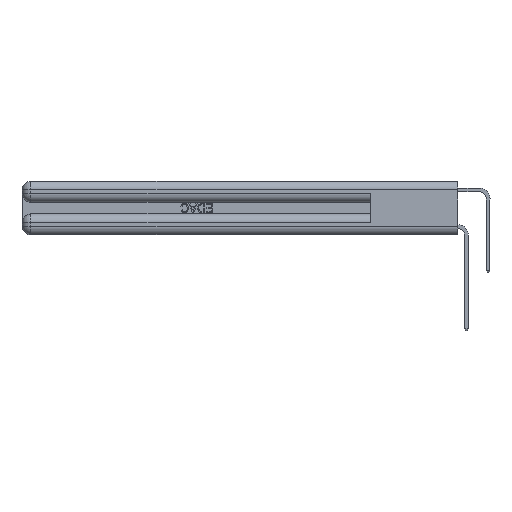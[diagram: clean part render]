
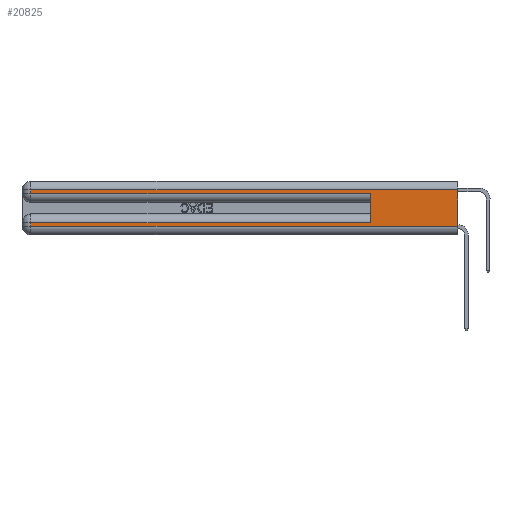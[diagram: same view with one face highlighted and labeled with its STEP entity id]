
A CAD part, left-side view. The second image highlights one B-rep face of the part: STEP entity #20825.
In plain terms, the highlighted planar face has unit normal (-1, 0, 0).
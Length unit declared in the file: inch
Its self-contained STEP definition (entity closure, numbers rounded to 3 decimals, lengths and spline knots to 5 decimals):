
#70 = LINE ( 'NONE', #30249, #3659 ) ;
#272 = DIRECTION ( 'NONE',  ( 0., 0., -1. ) ) ;
#492 = CARTESIAN_POINT ( 'NONE',  ( 0., 0., 0.37 ) ) ;
#1123 = LINE ( 'NONE', #13394, #12926 ) ;
#1516 = VECTOR ( 'NONE', #16111, 39.37008 ) ;
#1933 = CARTESIAN_POINT ( 'NONE',  ( 0., 0., 0.285 ) ) ;
#1957 = CARTESIAN_POINT ( 'NONE',  ( 0., 0., 0.37 ) ) ;
#2993 = DIRECTION ( 'NONE',  ( 0., 0., 1. ) ) ;
#3484 = CARTESIAN_POINT ( 'NONE',  ( 0., 0., 0.31 ) ) ;
#3612 = CARTESIAN_POINT ( 'NONE',  ( 0., 0., 0.06 ) ) ;
#3659 = VECTOR ( 'NONE', #2993, 39.37008 ) ;
#4809 = VECTOR ( 'NONE', #12495, 39.37008 ) ;
#4818 = EDGE_CURVE ( 'NONE', #23546, #12171, #24266, .T. ) ;
#5651 = VECTOR ( 'NONE', #6399, 39.37008 ) ;
#6399 = DIRECTION ( 'NONE',  ( 0., 1., 0. ) ) ;
#8438 = EDGE_CURVE ( 'NONE', #11112, #12171, #9797, .T. ) ;
#8594 = CARTESIAN_POINT ( 'NONE',  ( 0., 2.94, 0.37 ) ) ;
#9797 = LINE ( 'NONE', #31076, #1516 ) ;
#10317 = DIRECTION ( 'NONE',  ( 0., 1., 0. ) ) ;
#10382 = ORIENTED_EDGE ( 'NONE', *, *, #24543, .T. ) ;
#10434 = VECTOR ( 'NONE', #10317, 39.37008 ) ;
#10583 = AXIS2_PLACEMENT_3D ( 'NONE', #1957, #25064, #27660 ) ;
#11105 = DIRECTION ( 'NONE',  ( 0., 0., -1. ) ) ;
#11112 = VERTEX_POINT ( 'NONE', #29518 ) ;
#12127 = ORIENTED_EDGE ( 'NONE', *, *, #8438, .T. ) ;
#12171 = VERTEX_POINT ( 'NONE', #3612 ) ;
#12495 = DIRECTION ( 'NONE',  ( 0., -1., 0. ) ) ;
#12529 = VERTEX_POINT ( 'NONE', #23239 ) ;
#12844 = CARTESIAN_POINT ( 'NONE',  ( 0., 0., 0.31 ) ) ;
#12926 = VECTOR ( 'NONE', #20945, 39.37008 ) ;
#13193 = LINE ( 'NONE', #31609, #5651 ) ;
#13394 = CARTESIAN_POINT ( 'NONE',  ( 0., 2.94, 0.37 ) ) ;
#13824 = VERTEX_POINT ( 'NONE', #28223 ) ;
#14473 = EDGE_CURVE ( 'NONE', #32614, #31608, #24224, .T. ) ;
#16111 = DIRECTION ( 'NONE',  ( 0., -1., 0. ) ) ;
#16263 = ORIENTED_EDGE ( 'NONE', *, *, #31083, .T. ) ;
#17183 = LINE ( 'NONE', #12844, #10434 ) ;
#17457 = CARTESIAN_POINT ( 'NONE',  ( 0., 0.6, 0.085 ) ) ;
#18349 = LINE ( 'NONE', #8594, #24308 ) ;
#19607 = CARTESIAN_POINT ( 'NONE',  ( 0., 2.94, 0.285 ) ) ;
#20077 = EDGE_LOOP ( 'NONE', ( #32800, #10382, #31444, #21080, #30496, #16263, #32505, #12127 ) ) ;
#20825 = ADVANCED_FACE ( 'NONE', ( #29544 ), #29819, .F. ) ;
#20945 = DIRECTION ( 'NONE',  ( 0., 0., -1. ) ) ;
#21017 = EDGE_CURVE ( 'NONE', #13824, #11112, #18349, .T. ) ;
#21080 = ORIENTED_EDGE ( 'NONE', *, *, #14473, .T. ) ;
#21081 = CARTESIAN_POINT ( 'NONE',  ( 0., 0.6, 0.285 ) ) ;
#23239 = CARTESIAN_POINT ( 'NONE',  ( 0., 2.94, 0.31 ) ) ;
#23546 = VERTEX_POINT ( 'NONE', #3484 ) ;
#24224 = LINE ( 'NONE', #1933, #4809 ) ;
#24266 = LINE ( 'NONE', #492, #24657 ) ;
#24308 = VECTOR ( 'NONE', #11105, 39.37008 ) ;
#24543 = EDGE_CURVE ( 'NONE', #23546, #12529, #17183, .T. ) ;
#24657 = VECTOR ( 'NONE', #272, 39.37008 ) ;
#25064 = DIRECTION ( 'NONE',  ( 1., 0., 0. ) ) ;
#25803 = EDGE_CURVE ( 'NONE', #26982, #31608, #70, .T. ) ;
#26982 = VERTEX_POINT ( 'NONE', #17457 ) ;
#27660 = DIRECTION ( 'NONE',  ( 0., 0., -1. ) ) ;
#28223 = CARTESIAN_POINT ( 'NONE',  ( 0., 2.94, 0.085 ) ) ;
#28963 = EDGE_CURVE ( 'NONE', #12529, #32614, #1123, .T. ) ;
#29518 = CARTESIAN_POINT ( 'NONE',  ( 0., 2.94, 0.06 ) ) ;
#29544 = FACE_OUTER_BOUND ( 'NONE', #20077, .T. ) ;
#29819 = PLANE ( 'NONE',  #10583 ) ;
#30249 = CARTESIAN_POINT ( 'NONE',  ( 0., 0.6, 0.145 ) ) ;
#30496 = ORIENTED_EDGE ( 'NONE', *, *, #25803, .F. ) ;
#31076 = CARTESIAN_POINT ( 'NONE',  ( 0., 0., 0.06 ) ) ;
#31083 = EDGE_CURVE ( 'NONE', #26982, #13824, #13193, .T. ) ;
#31444 = ORIENTED_EDGE ( 'NONE', *, *, #28963, .T. ) ;
#31608 = VERTEX_POINT ( 'NONE', #21081 ) ;
#31609 = CARTESIAN_POINT ( 'NONE',  ( 0., 0., 0.085 ) ) ;
#32505 = ORIENTED_EDGE ( 'NONE', *, *, #21017, .T. ) ;
#32614 = VERTEX_POINT ( 'NONE', #19607 ) ;
#32800 = ORIENTED_EDGE ( 'NONE', *, *, #4818, .F. ) ;
